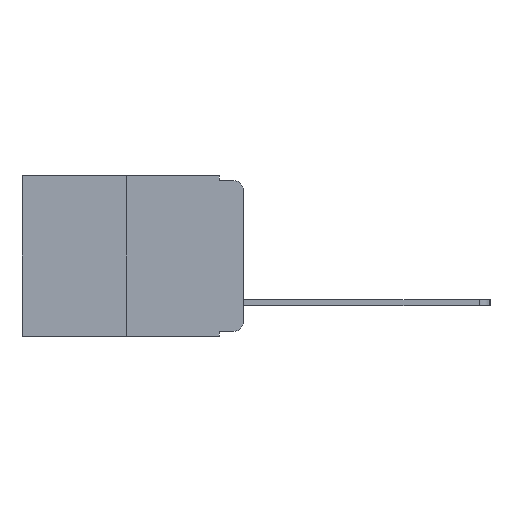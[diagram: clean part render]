
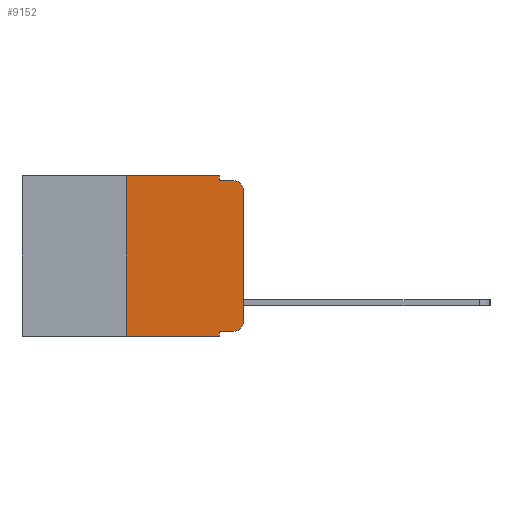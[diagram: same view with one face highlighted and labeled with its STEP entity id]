
A CAD part, left-side view. The second image highlights one B-rep face of the part: STEP entity #9152.
In plain terms, the highlighted planar face has unit normal (-1, 0, 0).
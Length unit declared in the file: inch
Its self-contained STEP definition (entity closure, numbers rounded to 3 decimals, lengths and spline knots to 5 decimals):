
#253 = CARTESIAN_POINT ( 'NONE',  ( 0., 0.051, -0.333 ) ) ;
#329 = CARTESIAN_POINT ( 'NONE',  ( 0., 0., -0.313 ) ) ;
#354 = EDGE_CURVE ( 'NONE', #655, #5559, #1913, .T. ) ;
#580 = DIRECTION ( 'NONE',  ( 0., 0., -1. ) ) ;
#655 = VERTEX_POINT ( 'NONE', #329 ) ;
#720 = CARTESIAN_POINT ( 'NONE',  ( 0., 0.25, 0. ) ) ;
#1077 = CARTESIAN_POINT ( 'NONE',  ( 0., 0.25, -0.343 ) ) ;
#1295 = AXIS2_PLACEMENT_3D ( 'NONE', #2063, #2061, #3802 ) ;
#1340 = CIRCLE ( 'NONE', #10369, 0.02 ) ;
#1642 = CARTESIAN_POINT ( 'NONE',  ( 0., 0.473, -0.343 ) ) ;
#1725 = VERTEX_POINT ( 'NONE', #10913 ) ;
#1913 = LINE ( 'NONE', #7726, #4105 ) ;
#2061 = DIRECTION ( 'NONE',  ( -1., 0., 0. ) ) ;
#2063 = CARTESIAN_POINT ( 'NONE',  ( 0., 0.02, -0.313 ) ) ;
#2302 = EDGE_LOOP ( 'NONE', ( #8333, #8266, #8226, #8103, #8072, #7903, #7526, #7547, #9618, #9236 ) ) ;
#2316 = EDGE_CURVE ( 'NONE', #3248, #3517, #3780, .T. ) ;
#2767 = VERTEX_POINT ( 'NONE', #5738 ) ;
#2827 = EDGE_CURVE ( 'NONE', #1725, #655, #9949, .T. ) ;
#3248 = VERTEX_POINT ( 'NONE', #1077 ) ;
#3376 = EDGE_CURVE ( 'NONE', #3248, #9229, #6034, .T. ) ;
#3399 = DIRECTION ( 'NONE',  ( -1., 0., 0. ) ) ;
#3505 = VECTOR ( 'NONE', #5840, 39.37008 ) ;
#3517 = VERTEX_POINT ( 'NONE', #720 ) ;
#3780 = LINE ( 'NONE', #3796, #7955 ) ;
#3796 = CARTESIAN_POINT ( 'NONE',  ( 0., 0.25, 0. ) ) ;
#3802 = DIRECTION ( 'NONE',  ( 0., 0., -1. ) ) ;
#3852 = EDGE_CURVE ( 'NONE', #2767, #4501, #3880, .T. ) ;
#3863 = DIRECTION ( 'NONE',  ( 0., 0., -1. ) ) ;
#3876 = VECTOR ( 'NONE', #11196, 39.37008 ) ;
#3880 = LINE ( 'NONE', #11176, #10323 ) ;
#4105 = VECTOR ( 'NONE', #10296, 39.37008 ) ;
#4226 = EDGE_CURVE ( 'NONE', #5344, #9229, #6295, .T. ) ;
#4315 = PLANE ( 'NONE',  #9590 ) ;
#4501 = VERTEX_POINT ( 'NONE', #9000 ) ;
#5223 = DIRECTION ( 'NONE',  ( 0., -1., 0. ) ) ;
#5231 = CARTESIAN_POINT ( 'NONE',  ( 0., 0.473, 0. ) ) ;
#5344 = VERTEX_POINT ( 'NONE', #11247 ) ;
#5559 = VERTEX_POINT ( 'NONE', #8130 ) ;
#5620 = VECTOR ( 'NONE', #11318, 39.37008 ) ;
#5694 = EDGE_CURVE ( 'NONE', #9213, #2767, #11380, .T. ) ;
#5738 = CARTESIAN_POINT ( 'NONE',  ( 0., 0.051, -0.01 ) ) ;
#5840 = DIRECTION ( 'NONE',  ( 0., -1., 0. ) ) ;
#6034 = LINE ( 'NONE', #1642, #10617 ) ;
#6132 = DIRECTION ( 'NONE',  ( 1., 0., 0. ) ) ;
#6175 = CARTESIAN_POINT ( 'NONE',  ( 0., 0.473, 0. ) ) ;
#6295 = LINE ( 'NONE', #6472, #3876 ) ;
#6472 = CARTESIAN_POINT ( 'NONE',  ( 0., 0.051, 0. ) ) ;
#6532 = CARTESIAN_POINT ( 'NONE',  ( 0., 0.051, 0. ) ) ;
#6608 = EDGE_CURVE ( 'NONE', #5559, #4501, #1340, .T. ) ;
#6797 = DIRECTION ( 'NONE',  ( 0., 0., 1. ) ) ;
#7101 = CARTESIAN_POINT ( 'NONE',  ( 0., 0.051, -0.343 ) ) ;
#7526 = ORIENTED_EDGE ( 'NONE', *, *, #3376, .T. ) ;
#7547 = ORIENTED_EDGE ( 'NONE', *, *, #4226, .F. ) ;
#7726 = CARTESIAN_POINT ( 'NONE',  ( 0., 0., 0. ) ) ;
#7903 = ORIENTED_EDGE ( 'NONE', *, *, #2316, .F. ) ;
#7955 = VECTOR ( 'NONE', #6797, 39.37008 ) ;
#8072 = ORIENTED_EDGE ( 'NONE', *, *, #9187, .F. ) ;
#8103 = ORIENTED_EDGE ( 'NONE', *, *, #5694, .F. ) ;
#8130 = CARTESIAN_POINT ( 'NONE',  ( 0., 0., -0.03 ) ) ;
#8221 = LINE ( 'NONE', #253, #3505 ) ;
#8226 = ORIENTED_EDGE ( 'NONE', *, *, #3852, .F. ) ;
#8266 = ORIENTED_EDGE ( 'NONE', *, *, #6608, .T. ) ;
#8333 = ORIENTED_EDGE ( 'NONE', *, *, #354, .T. ) ;
#8347 = EDGE_CURVE ( 'NONE', #5344, #1725, #8221, .T. ) ;
#8705 = CARTESIAN_POINT ( 'NONE',  ( 0., 0.02, -0.03 ) ) ;
#9000 = CARTESIAN_POINT ( 'NONE',  ( 0., 0.02, -0.01 ) ) ;
#9152 = ADVANCED_FACE ( 'NONE', ( #10763 ), #4315, .F. ) ;
#9187 = EDGE_CURVE ( 'NONE', #3517, #9213, #10206, .T. ) ;
#9213 = VERTEX_POINT ( 'NONE', #10520 ) ;
#9229 = VERTEX_POINT ( 'NONE', #7101 ) ;
#9236 = ORIENTED_EDGE ( 'NONE', *, *, #2827, .T. ) ;
#9260 = DIRECTION ( 'NONE',  ( 0., -1., 0. ) ) ;
#9563 = DIRECTION ( 'NONE',  ( 0., 0., -1. ) ) ;
#9590 = AXIS2_PLACEMENT_3D ( 'NONE', #5231, #6132, #580 ) ;
#9618 = ORIENTED_EDGE ( 'NONE', *, *, #8347, .T. ) ;
#9949 = CIRCLE ( 'NONE', #1295, 0.02 ) ;
#10206 = LINE ( 'NONE', #6175, #5620 ) ;
#10296 = DIRECTION ( 'NONE',  ( 0., 0., 1. ) ) ;
#10323 = VECTOR ( 'NONE', #5223, 39.37008 ) ;
#10369 = AXIS2_PLACEMENT_3D ( 'NONE', #8705, #3399, #9563 ) ;
#10520 = CARTESIAN_POINT ( 'NONE',  ( 0., 0.051, 0. ) ) ;
#10617 = VECTOR ( 'NONE', #9260, 39.37008 ) ;
#10763 = FACE_OUTER_BOUND ( 'NONE', #2302, .T. ) ;
#10913 = CARTESIAN_POINT ( 'NONE',  ( 0., 0.02, -0.333 ) ) ;
#11113 = VECTOR ( 'NONE', #3863, 39.37008 ) ;
#11176 = CARTESIAN_POINT ( 'NONE',  ( 0., 0.051, -0.01 ) ) ;
#11196 = DIRECTION ( 'NONE',  ( 0., 0., -1. ) ) ;
#11247 = CARTESIAN_POINT ( 'NONE',  ( 0., 0.051, -0.333 ) ) ;
#11318 = DIRECTION ( 'NONE',  ( 0., -1., 0. ) ) ;
#11380 = LINE ( 'NONE', #6532, #11113 ) ;
